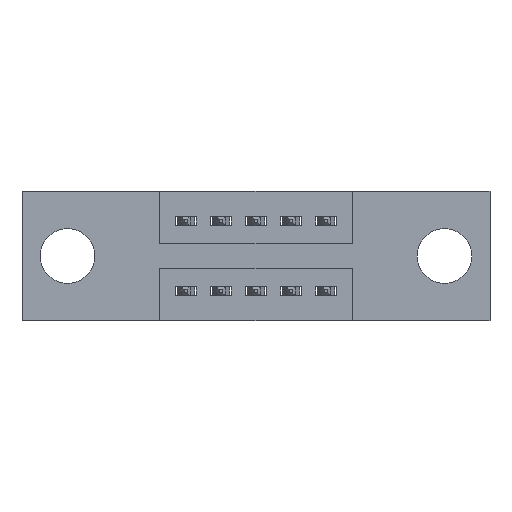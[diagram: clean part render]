
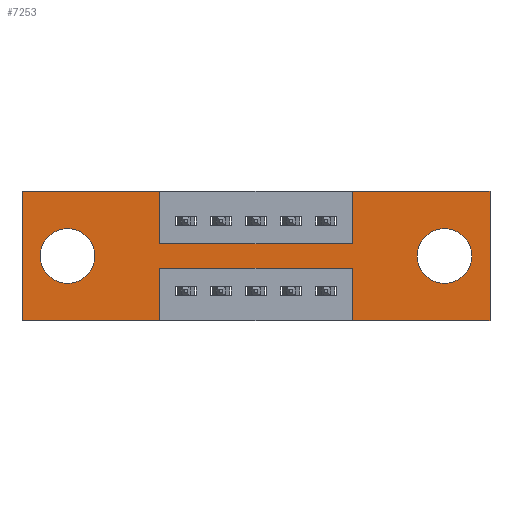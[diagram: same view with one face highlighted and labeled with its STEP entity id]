
A CAD part, front view. The second image highlights one B-rep face of the part: STEP entity #7253.
In plain terms, the highlighted planar face has unit normal (0, -1, 0).
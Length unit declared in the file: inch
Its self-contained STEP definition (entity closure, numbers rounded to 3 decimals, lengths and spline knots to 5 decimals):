
#8 = DIRECTION ( 'NONE',  ( -1., 0., 0. ) ) ;
#19 = EDGE_CURVE ( 'NONE', #8263, #2362, #2370, .T. ) ;
#91 = CARTESIAN_POINT ( 'NONE',  ( 0., 0., 0. ) ) ;
#129 = LINE ( 'NONE', #4307, #7148 ) ;
#185 = DIRECTION ( 'NONE',  ( 0., 0., -1. ) ) ;
#198 = CARTESIAN_POINT ( 'NONE',  ( 0., 0., -0.37 ) ) ;
#398 = ORIENTED_EDGE ( 'NONE', *, *, #6303, .F. ) ;
#581 = ORIENTED_EDGE ( 'NONE', *, *, #8709, .F. ) ;
#609 = DIRECTION ( 'NONE',  ( 0., 0., 1. ) ) ;
#726 = DIRECTION ( 'NONE',  ( 0., 0., -1. ) ) ;
#768 = LINE ( 'NONE', #198, #6088 ) ;
#903 = CARTESIAN_POINT ( 'NONE',  ( 0.3925, 0., -0.37 ) ) ;
#1023 = DIRECTION ( 'NONE',  ( 1., 0., 0. ) ) ;
#1054 = ORIENTED_EDGE ( 'NONE', *, *, #5660, .T. ) ;
#1111 = EDGE_CURVE ( 'NONE', #6206, #1409, #1423, .T. ) ;
#1168 = CARTESIAN_POINT ( 'NONE',  ( 0.9425, 0., 0. ) ) ;
#1289 = ORIENTED_EDGE ( 'NONE', *, *, #6022, .F. ) ;
#1386 = CIRCLE ( 'NONE', #7290, 0.078 ) ;
#1409 = VERTEX_POINT ( 'NONE', #5471 ) ;
#1423 = LINE ( 'NONE', #3030, #2058 ) ;
#1461 = LINE ( 'NONE', #8787, #4431 ) ;
#1494 = DIRECTION ( 'NONE',  ( 0., 0., 1. ) ) ;
#1749 = DIRECTION ( 'NONE',  ( 0., 1., 0. ) ) ;
#1772 = DIRECTION ( 'NONE',  ( 0., 0., -1. ) ) ;
#1922 = FACE_BOUND ( 'NONE', #2477, .T. ) ;
#1950 = CARTESIAN_POINT ( 'NONE',  ( 0.3925, 0., -0.22 ) ) ;
#2058 = VECTOR ( 'NONE', #185, 39.37008 ) ;
#2087 = ORIENTED_EDGE ( 'NONE', *, *, #6542, .F. ) ;
#2199 = ORIENTED_EDGE ( 'NONE', *, *, #5987, .F. ) ;
#2260 = ORIENTED_EDGE ( 'NONE', *, *, #2867, .T. ) ;
#2362 = VERTEX_POINT ( 'NONE', #5294 ) ;
#2370 = LINE ( 'NONE', #2509, #6347 ) ;
#2395 = VERTEX_POINT ( 'NONE', #2423 ) ;
#2423 = CARTESIAN_POINT ( 'NONE',  ( 0., 0., -0.37 ) ) ;
#2477 = EDGE_LOOP ( 'NONE', ( #1054, #6543 ) ) ;
#2502 = CARTESIAN_POINT ( 'NONE',  ( 1.335, 0., 0. ) ) ;
#2509 = CARTESIAN_POINT ( 'NONE',  ( 0., 0., 0. ) ) ;
#2514 = AXIS2_PLACEMENT_3D ( 'NONE', #5995, #1749, #6093 ) ;
#2587 = FACE_BOUND ( 'NONE', #7810, .T. ) ;
#2632 = EDGE_LOOP ( 'NONE', ( #2872, #2087, #581, #6689, #3778, #5147, #2199, #1289, #398, #9249, #6057, #5658 ) ) ;
#2867 = EDGE_CURVE ( 'NONE', #3537, #5854, #1386, .T. ) ;
#2872 = ORIENTED_EDGE ( 'NONE', *, *, #8714, .F. ) ;
#2922 = LINE ( 'NONE', #4386, #9125 ) ;
#2928 = VERTEX_POINT ( 'NONE', #1950 ) ;
#2936 = LINE ( 'NONE', #7225, #4134 ) ;
#3030 = CARTESIAN_POINT ( 'NONE',  ( 1.335, 0., 0. ) ) ;
#3093 = AXIS2_PLACEMENT_3D ( 'NONE', #8627, #5176, #726 ) ;
#3176 = LINE ( 'NONE', #8947, #7768 ) ;
#3336 = VERTEX_POINT ( 'NONE', #1168 ) ;
#3391 = FACE_OUTER_BOUND ( 'NONE', #2632, .T. ) ;
#3473 = LINE ( 'NONE', #4940, #7461 ) ;
#3525 = ORIENTED_EDGE ( 'NONE', *, *, #8112, .T. ) ;
#3537 = VERTEX_POINT ( 'NONE', #6459 ) ;
#3593 = DIRECTION ( 'NONE',  ( 1., 0., 0. ) ) ;
#3777 = DIRECTION ( 'NONE',  ( 0., 0., 1. ) ) ;
#3778 = ORIENTED_EDGE ( 'NONE', *, *, #1111, .F. ) ;
#3947 = EDGE_CURVE ( 'NONE', #4953, #2395, #768, .T. ) ;
#4046 = VERTEX_POINT ( 'NONE', #6763 ) ;
#4073 = EDGE_CURVE ( 'NONE', #3336, #6206, #3176, .T. ) ;
#4134 = VECTOR ( 'NONE', #4440, 39.37008 ) ;
#4187 = CIRCLE ( 'NONE', #4343, 0.078 ) ;
#4212 = CARTESIAN_POINT ( 'NONE',  ( 0.13, 0., -0.185 ) ) ;
#4307 = CARTESIAN_POINT ( 'NONE',  ( 0.3925, 0., -0.15 ) ) ;
#4332 = CARTESIAN_POINT ( 'NONE',  ( 0.3925, 0., -0.15 ) ) ;
#4343 = AXIS2_PLACEMENT_3D ( 'NONE', #6613, #5118, #6654 ) ;
#4386 = CARTESIAN_POINT ( 'NONE',  ( 0.3925, 0., -0.22 ) ) ;
#4423 = EDGE_CURVE ( 'NONE', #7591, #8828, #7493, .T. ) ;
#4431 = VECTOR ( 'NONE', #3777, 39.37008 ) ;
#4440 = DIRECTION ( 'NONE',  ( -1., 0., 0. ) ) ;
#4556 = VERTEX_POINT ( 'NONE', #6364 ) ;
#4849 = VECTOR ( 'NONE', #1494, 39.37008 ) ;
#4940 = CARTESIAN_POINT ( 'NONE',  ( 0., 0., 0. ) ) ;
#4953 = VERTEX_POINT ( 'NONE', #9165 ) ;
#5118 = DIRECTION ( 'NONE',  ( 0., 1., 0. ) ) ;
#5147 = ORIENTED_EDGE ( 'NONE', *, *, #4073, .F. ) ;
#5176 = DIRECTION ( 'NONE',  ( 0., -1., 0. ) ) ;
#5294 = CARTESIAN_POINT ( 'NONE',  ( 0.3925, 0., 0. ) ) ;
#5471 = CARTESIAN_POINT ( 'NONE',  ( 1.335, 0., -0.37 ) ) ;
#5559 = CARTESIAN_POINT ( 'NONE',  ( 0.9425, 0., -0.15 ) ) ;
#5599 = DIRECTION ( 'NONE',  ( 0., 0., -1. ) ) ;
#5658 = ORIENTED_EDGE ( 'NONE', *, *, #3947, .F. ) ;
#5660 = EDGE_CURVE ( 'NONE', #8828, #7591, #4187, .T. ) ;
#5661 = DIRECTION ( 'NONE',  ( 0., 0., 1. ) ) ;
#5730 = PLANE ( 'NONE',  #3093 ) ;
#5854 = VERTEX_POINT ( 'NONE', #7762 ) ;
#5953 = EDGE_CURVE ( 'NONE', #1409, #4556, #2936, .T. ) ;
#5987 = EDGE_CURVE ( 'NONE', #6772, #3336, #1461, .T. ) ;
#5995 = CARTESIAN_POINT ( 'NONE',  ( 1.205, 0., -0.185 ) ) ;
#6022 = EDGE_CURVE ( 'NONE', #7374, #6772, #129, .T. ) ;
#6057 = ORIENTED_EDGE ( 'NONE', *, *, #7182, .F. ) ;
#6088 = VECTOR ( 'NONE', #8, 39.37008 ) ;
#6093 = DIRECTION ( 'NONE',  ( 0., 0., -1. ) ) ;
#6195 = AXIS2_PLACEMENT_3D ( 'NONE', #6370, #8651, #5661 ) ;
#6206 = VERTEX_POINT ( 'NONE', #2502 ) ;
#6303 = EDGE_CURVE ( 'NONE', #2362, #7374, #9118, .T. ) ;
#6325 = DIRECTION ( 'NONE',  ( 0., 1., 0. ) ) ;
#6347 = VECTOR ( 'NONE', #1023, 39.37008 ) ;
#6364 = CARTESIAN_POINT ( 'NONE',  ( 0.9425, 0., -0.37 ) ) ;
#6370 = CARTESIAN_POINT ( 'NONE',  ( 0.13, 0., -0.185 ) ) ;
#6459 = CARTESIAN_POINT ( 'NONE',  ( 0.13, 0., -0.107 ) ) ;
#6542 = EDGE_CURVE ( 'NONE', #4046, #2928, #2922, .T. ) ;
#6543 = ORIENTED_EDGE ( 'NONE', *, *, #4423, .T. ) ;
#6613 = CARTESIAN_POINT ( 'NONE',  ( 1.205, 0., -0.185 ) ) ;
#6654 = DIRECTION ( 'NONE',  ( 0., 0., -1. ) ) ;
#6689 = ORIENTED_EDGE ( 'NONE', *, *, #5953, .F. ) ;
#6763 = CARTESIAN_POINT ( 'NONE',  ( 0.9425, 0., -0.22 ) ) ;
#6772 = VERTEX_POINT ( 'NONE', #5559 ) ;
#7148 = VECTOR ( 'NONE', #3593, 39.37008 ) ;
#7182 = EDGE_CURVE ( 'NONE', #2395, #8263, #3473, .T. ) ;
#7225 = CARTESIAN_POINT ( 'NONE',  ( 0., 0., -0.37 ) ) ;
#7253 = ADVANCED_FACE ( 'NONE', ( #1922, #2587, #3391 ), #5730, .T. ) ;
#7263 = DIRECTION ( 'NONE',  ( -1., 0., 0. ) ) ;
#7290 = AXIS2_PLACEMENT_3D ( 'NONE', #4212, #6325, #609 ) ;
#7374 = VERTEX_POINT ( 'NONE', #4332 ) ;
#7391 = LINE ( 'NONE', #903, #9077 ) ;
#7461 = VECTOR ( 'NONE', #9198, 39.37008 ) ;
#7493 = CIRCLE ( 'NONE', #2514, 0.078 ) ;
#7591 = VERTEX_POINT ( 'NONE', #8476 ) ;
#7751 = CARTESIAN_POINT ( 'NONE',  ( 0.3925, 0., 0. ) ) ;
#7762 = CARTESIAN_POINT ( 'NONE',  ( 0.13, 0., -0.263 ) ) ;
#7768 = VECTOR ( 'NONE', #8242, 39.37008 ) ;
#7810 = EDGE_LOOP ( 'NONE', ( #2260, #3525 ) ) ;
#7823 = CARTESIAN_POINT ( 'NONE',  ( 1.205, 0., -0.107 ) ) ;
#7990 = CARTESIAN_POINT ( 'NONE',  ( 0.9425, 0., -0.37 ) ) ;
#8112 = EDGE_CURVE ( 'NONE', #5854, #3537, #8170, .T. ) ;
#8170 = CIRCLE ( 'NONE', #6195, 0.078 ) ;
#8242 = DIRECTION ( 'NONE',  ( 1., 0., 0. ) ) ;
#8249 = LINE ( 'NONE', #7990, #4849 ) ;
#8263 = VERTEX_POINT ( 'NONE', #91 ) ;
#8476 = CARTESIAN_POINT ( 'NONE',  ( 1.205, 0., -0.263 ) ) ;
#8627 = CARTESIAN_POINT ( 'NONE',  ( 0., 0., -0.37 ) ) ;
#8651 = DIRECTION ( 'NONE',  ( 0., 1., 0. ) ) ;
#8664 = VECTOR ( 'NONE', #5599, 39.37008 ) ;
#8709 = EDGE_CURVE ( 'NONE', #4556, #4046, #8249, .T. ) ;
#8714 = EDGE_CURVE ( 'NONE', #2928, #4953, #7391, .T. ) ;
#8787 = CARTESIAN_POINT ( 'NONE',  ( 0.9425, 0., 0. ) ) ;
#8828 = VERTEX_POINT ( 'NONE', #7823 ) ;
#8947 = CARTESIAN_POINT ( 'NONE',  ( 0., 0., 0. ) ) ;
#9077 = VECTOR ( 'NONE', #1772, 39.37008 ) ;
#9118 = LINE ( 'NONE', #7751, #8664 ) ;
#9125 = VECTOR ( 'NONE', #7263, 39.37008 ) ;
#9165 = CARTESIAN_POINT ( 'NONE',  ( 0.3925, 0., -0.37 ) ) ;
#9198 = DIRECTION ( 'NONE',  ( 0., 0., 1. ) ) ;
#9249 = ORIENTED_EDGE ( 'NONE', *, *, #19, .F. ) ;
